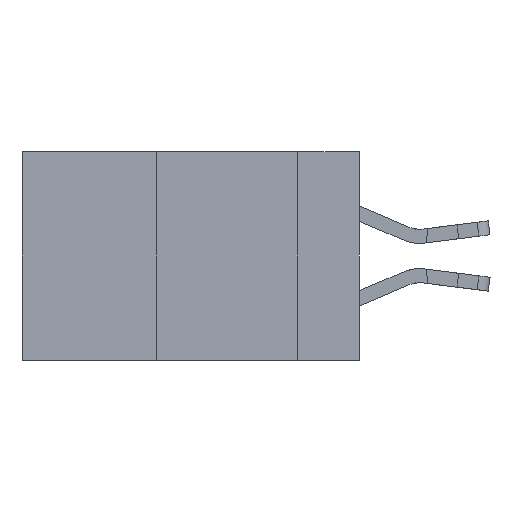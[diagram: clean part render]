
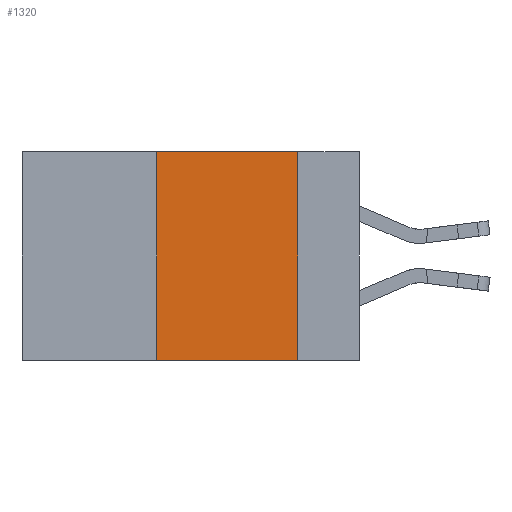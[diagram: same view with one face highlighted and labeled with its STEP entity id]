
A CAD part, left-side view. The second image highlights one B-rep face of the part: STEP entity #1320.
In plain terms, the highlighted planar face has unit normal (-1, 0, 0).
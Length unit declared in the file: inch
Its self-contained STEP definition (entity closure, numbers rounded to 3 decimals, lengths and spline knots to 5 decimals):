
#1320 = ADVANCED_FACE ( 'NONE', ( #11687 ), #8645, .F. ) ;
#1607 = ORIENTED_EDGE ( 'NONE', *, *, #10043, .F. ) ;
#2420 = LINE ( 'NONE', #3056, #3997 ) ;
#2535 = EDGE_CURVE ( 'NONE', #23839, #3085, #10157, .T. ) ;
#2711 = DIRECTION ( 'NONE',  ( 0., 0., 1. ) ) ;
#2874 = LINE ( 'NONE', #20985, #25056 ) ;
#3056 = CARTESIAN_POINT ( 'NONE',  ( 0., 0.36, 0. ) ) ;
#3085 = VERTEX_POINT ( 'NONE', #21151 ) ;
#3500 = CARTESIAN_POINT ( 'NONE',  ( 0., 0.11, 0. ) ) ;
#3997 = VECTOR ( 'NONE', #2711, 39.37008 ) ;
#4687 = CARTESIAN_POINT ( 'NONE',  ( 0., 0.36, 0. ) ) ;
#5881 = EDGE_LOOP ( 'NONE', ( #10734, #11792, #1607, #15082 ) ) ;
#6088 = AXIS2_PLACEMENT_3D ( 'NONE', #12286, #22234, #8561 ) ;
#6178 = CARTESIAN_POINT ( 'NONE',  ( 0., 0.36, -0.37 ) ) ;
#8561 = DIRECTION ( 'NONE',  ( 0., 0., -1. ) ) ;
#8645 = PLANE ( 'NONE',  #6088 ) ;
#8807 = VERTEX_POINT ( 'NONE', #4687 ) ;
#10043 = EDGE_CURVE ( 'NONE', #23839, #8807, #2420, .T. ) ;
#10157 = LINE ( 'NONE', #14403, #14158 ) ;
#10694 = DIRECTION ( 'NONE',  ( 0., -1., 0. ) ) ;
#10734 = ORIENTED_EDGE ( 'NONE', *, *, #16592, .F. ) ;
#11687 = FACE_OUTER_BOUND ( 'NONE', #5881, .T. ) ;
#11792 = ORIENTED_EDGE ( 'NONE', *, *, #25432, .F. ) ;
#12286 = CARTESIAN_POINT ( 'NONE',  ( 0., 0.6, 0. ) ) ;
#12760 = VERTEX_POINT ( 'NONE', #3500 ) ;
#13064 = LINE ( 'NONE', #23087, #22275 ) ;
#14158 = VECTOR ( 'NONE', #10694, 39.37008 ) ;
#14403 = CARTESIAN_POINT ( 'NONE',  ( 0., 0.6, -0.37 ) ) ;
#15082 = ORIENTED_EDGE ( 'NONE', *, *, #2535, .T. ) ;
#15178 = DIRECTION ( 'NONE',  ( 0., 0., -1. ) ) ;
#16592 = EDGE_CURVE ( 'NONE', #12760, #3085, #13064, .T. ) ;
#20985 = CARTESIAN_POINT ( 'NONE',  ( 0., 0.6, 0. ) ) ;
#21151 = CARTESIAN_POINT ( 'NONE',  ( 0., 0.11, -0.37 ) ) ;
#22234 = DIRECTION ( 'NONE',  ( 1., 0., 0. ) ) ;
#22275 = VECTOR ( 'NONE', #15178, 39.37008 ) ;
#23087 = CARTESIAN_POINT ( 'NONE',  ( 0., 0.11, 0. ) ) ;
#23128 = DIRECTION ( 'NONE',  ( 0., -1., 0. ) ) ;
#23839 = VERTEX_POINT ( 'NONE', #6178 ) ;
#25056 = VECTOR ( 'NONE', #23128, 39.37008 ) ;
#25432 = EDGE_CURVE ( 'NONE', #8807, #12760, #2874, .T. ) ;
